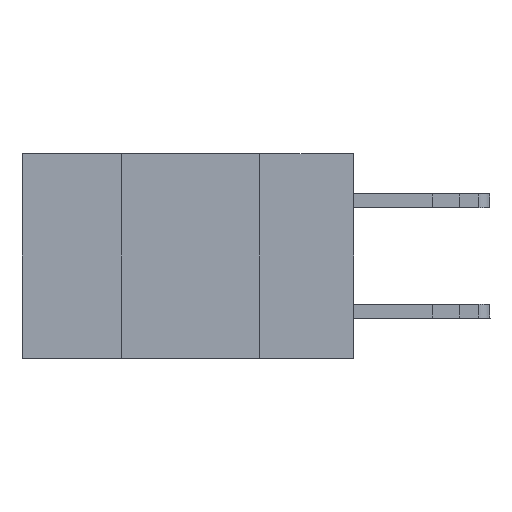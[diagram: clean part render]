
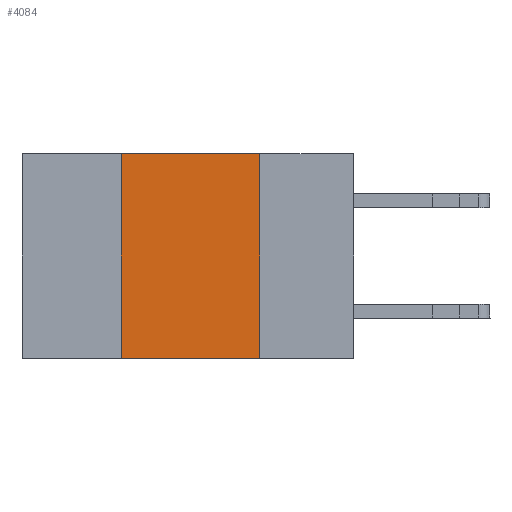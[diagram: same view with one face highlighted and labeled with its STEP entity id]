
A CAD part, left-side view. The second image highlights one B-rep face of the part: STEP entity #4084.
In plain terms, the highlighted planar face has unit normal (-1, 0, 0).
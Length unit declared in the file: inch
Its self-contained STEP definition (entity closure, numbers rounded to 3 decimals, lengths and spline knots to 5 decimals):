
#65 = VERTEX_POINT ( 'NONE', #4430 ) ;
#963 = VERTEX_POINT ( 'NONE', #1585 ) ;
#1585 = CARTESIAN_POINT ( 'NONE',  ( 0., 0.42, -0.37 ) ) ;
#2728 = LINE ( 'NONE', #16973, #16433 ) ;
#2755 = DIRECTION ( 'NONE',  ( 0., 0., 1. ) ) ;
#2850 = CARTESIAN_POINT ( 'NONE',  ( 0., 0.17, 0. ) ) ;
#3818 = VECTOR ( 'NONE', #11985, 39.37008 ) ;
#4084 = ADVANCED_FACE ( 'NONE', ( #8151 ), #16812, .F. ) ;
#4430 = CARTESIAN_POINT ( 'NONE',  ( 0., 0.17, -0.37 ) ) ;
#5162 = EDGE_LOOP ( 'NONE', ( #10941, #12030, #23058, #22311 ) ) ;
#5758 = VECTOR ( 'NONE', #12716, 39.37008 ) ;
#6347 = LINE ( 'NONE', #10979, #5758 ) ;
#8151 = FACE_OUTER_BOUND ( 'NONE', #5162, .T. ) ;
#8373 = EDGE_CURVE ( 'NONE', #963, #65, #18346, .T. ) ;
#8754 = LINE ( 'NONE', #2850, #3818 ) ;
#9877 = DIRECTION ( 'NONE',  ( 1., 0., 0. ) ) ;
#9894 = VERTEX_POINT ( 'NONE', #13825 ) ;
#10941 = ORIENTED_EDGE ( 'NONE', *, *, #18969, .F. ) ;
#10979 = CARTESIAN_POINT ( 'NONE',  ( 0., 0.6, 0. ) ) ;
#11985 = DIRECTION ( 'NONE',  ( 0., 0., -1. ) ) ;
#12030 = ORIENTED_EDGE ( 'NONE', *, *, #13004, .F. ) ;
#12716 = DIRECTION ( 'NONE',  ( 0., -1., 0. ) ) ;
#12861 = DIRECTION ( 'NONE',  ( 0., -1., 0. ) ) ;
#13004 = EDGE_CURVE ( 'NONE', #9894, #21669, #6347, .T. ) ;
#13739 = CARTESIAN_POINT ( 'NONE',  ( 0., 0.17, 0. ) ) ;
#13825 = CARTESIAN_POINT ( 'NONE',  ( 0., 0.42, 0. ) ) ;
#14600 = AXIS2_PLACEMENT_3D ( 'NONE', #20271, #9877, #21983 ) ;
#16433 = VECTOR ( 'NONE', #2755, 39.37008 ) ;
#16695 = EDGE_CURVE ( 'NONE', #963, #9894, #2728, .T. ) ;
#16812 = PLANE ( 'NONE',  #14600 ) ;
#16973 = CARTESIAN_POINT ( 'NONE',  ( 0., 0.42, 0. ) ) ;
#18346 = LINE ( 'NONE', #19800, #22325 ) ;
#18969 = EDGE_CURVE ( 'NONE', #21669, #65, #8754, .T. ) ;
#19800 = CARTESIAN_POINT ( 'NONE',  ( 0., 0.6, -0.37 ) ) ;
#20271 = CARTESIAN_POINT ( 'NONE',  ( 0., 0.6, 0. ) ) ;
#21669 = VERTEX_POINT ( 'NONE', #13739 ) ;
#21983 = DIRECTION ( 'NONE',  ( 0., 0., -1. ) ) ;
#22311 = ORIENTED_EDGE ( 'NONE', *, *, #8373, .T. ) ;
#22325 = VECTOR ( 'NONE', #12861, 39.37008 ) ;
#23058 = ORIENTED_EDGE ( 'NONE', *, *, #16695, .F. ) ;
